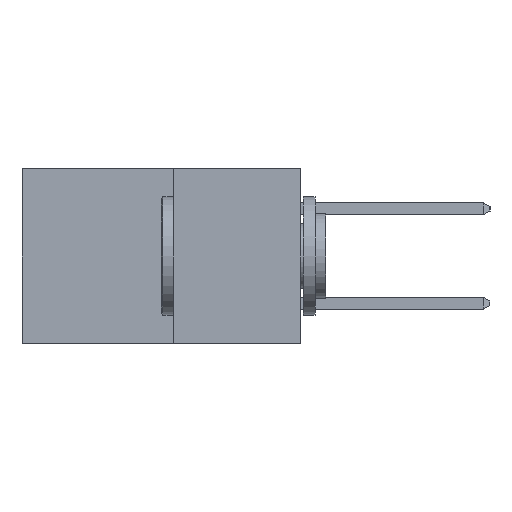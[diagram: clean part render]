
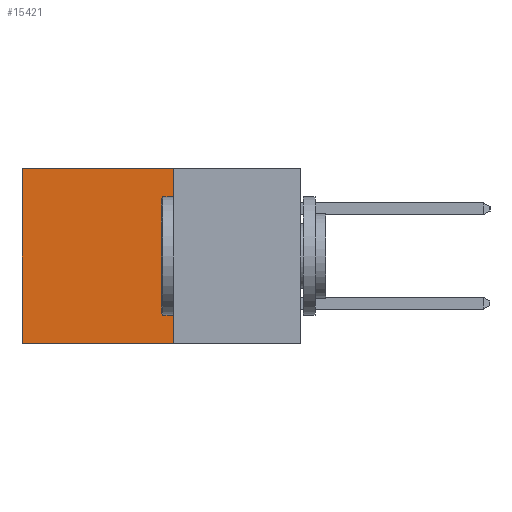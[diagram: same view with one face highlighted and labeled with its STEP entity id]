
A CAD part, left-side view. The second image highlights one B-rep face of the part: STEP entity #15421.
In plain terms, the highlighted planar face has unit normal (-1, 0, 0).
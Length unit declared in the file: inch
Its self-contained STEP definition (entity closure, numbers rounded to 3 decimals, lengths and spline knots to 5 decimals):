
#505 = PLANE ( 'NONE',  #8508 ) ;
#1268 = VECTOR ( 'NONE', #24907, 39.37008 ) ;
#2505 = DIRECTION ( 'NONE',  ( 0., 1., 0. ) ) ;
#2696 = VECTOR ( 'NONE', #28291, 39.37008 ) ;
#2861 = VERTEX_POINT ( 'NONE', #9236 ) ;
#4193 = EDGE_CURVE ( 'NONE', #2861, #16898, #12399, .T. ) ;
#5119 = CARTESIAN_POINT ( 'NONE',  ( 0.277, 0.27, -0.37 ) ) ;
#5144 = ORIENTED_EDGE ( 'NONE', *, *, #16651, .T. ) ;
#5671 = CARTESIAN_POINT ( 'NONE',  ( 0.277, 0.27, 0. ) ) ;
#5837 = CARTESIAN_POINT ( 'NONE',  ( 0.277, 0.27, -0.37 ) ) ;
#6336 = VECTOR ( 'NONE', #2505, 39.37008 ) ;
#7117 = VERTEX_POINT ( 'NONE', #5671 ) ;
#7364 = LINE ( 'NONE', #17966, #1268 ) ;
#7423 = DIRECTION ( 'NONE',  ( 1., 0., 0. ) ) ;
#8473 = ORIENTED_EDGE ( 'NONE', *, *, #9501, .T. ) ;
#8508 = AXIS2_PLACEMENT_3D ( 'NONE', #5119, #7423, #23457 ) ;
#9236 = CARTESIAN_POINT ( 'NONE',  ( 0.277, 0.27, -0.37 ) ) ;
#9501 = EDGE_CURVE ( 'NONE', #7117, #29316, #7364, .T. ) ;
#10202 = EDGE_CURVE ( 'NONE', #7117, #2861, #24546, .T. ) ;
#12399 = LINE ( 'NONE', #5837, #6336 ) ;
#14909 = LINE ( 'NONE', #25926, #2696 ) ;
#15421 = ADVANCED_FACE ( 'NONE', ( #24321 ), #505, .F. ) ;
#16651 = EDGE_CURVE ( 'NONE', #29316, #16898, #14909, .T. ) ;
#16898 = VERTEX_POINT ( 'NONE', #28968 ) ;
#17711 = ORIENTED_EDGE ( 'NONE', *, *, #10202, .F. ) ;
#17966 = CARTESIAN_POINT ( 'NONE',  ( 0.277, 0.27, 0. ) ) ;
#18422 = VECTOR ( 'NONE', #18772, 39.37008 ) ;
#18650 = EDGE_LOOP ( 'NONE', ( #5144, #29620, #17711, #8473 ) ) ;
#18772 = DIRECTION ( 'NONE',  ( 0., 0., -1. ) ) ;
#19879 = CARTESIAN_POINT ( 'NONE',  ( 0.277, 0.59, 0. ) ) ;
#23457 = DIRECTION ( 'NONE',  ( 0., 0., -1. ) ) ;
#24321 = FACE_OUTER_BOUND ( 'NONE', #18650, .T. ) ;
#24546 = LINE ( 'NONE', #25650, #18422 ) ;
#24907 = DIRECTION ( 'NONE',  ( 0., 1., 0. ) ) ;
#25650 = CARTESIAN_POINT ( 'NONE',  ( 0.277, 0.27, -0.37 ) ) ;
#25926 = CARTESIAN_POINT ( 'NONE',  ( 0.277, 0.59, -0.37 ) ) ;
#28291 = DIRECTION ( 'NONE',  ( 0., 0., -1. ) ) ;
#28968 = CARTESIAN_POINT ( 'NONE',  ( 0.277, 0.59, -0.37 ) ) ;
#29316 = VERTEX_POINT ( 'NONE', #19879 ) ;
#29620 = ORIENTED_EDGE ( 'NONE', *, *, #4193, .F. ) ;
